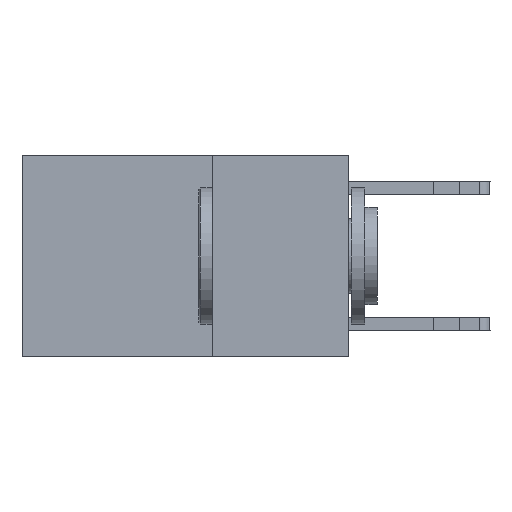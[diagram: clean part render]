
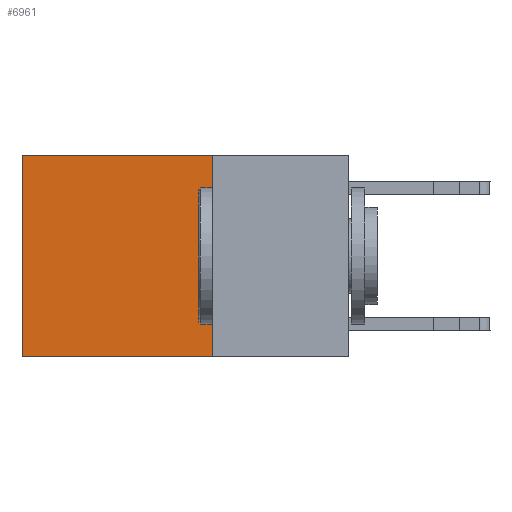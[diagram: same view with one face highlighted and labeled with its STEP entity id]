
A CAD part, left-side view. The second image highlights one B-rep face of the part: STEP entity #6961.
In plain terms, the highlighted planar face has unit normal (-1, 0, 0).
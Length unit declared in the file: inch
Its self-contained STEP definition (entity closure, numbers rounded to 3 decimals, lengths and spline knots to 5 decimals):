
#176 = AXIS2_PLACEMENT_3D ( 'NONE', #13911, #6382, #18770 ) ;
#232 = DIRECTION ( 'NONE',  ( 0., 0., -1. ) ) ;
#1264 = LINE ( 'NONE', #7343, #15404 ) ;
#1530 = LINE ( 'NONE', #12362, #6973 ) ;
#3976 = CARTESIAN_POINT ( 'NONE',  ( 0.2625, 0.6, 0. ) ) ;
#4156 = DIRECTION ( 'NONE',  ( 0., 1., 0. ) ) ;
#4174 = DIRECTION ( 'NONE',  ( 0., 0., -1. ) ) ;
#4298 = VERTEX_POINT ( 'NONE', #5183 ) ;
#4659 = ORIENTED_EDGE ( 'NONE', *, *, #18073, .F. ) ;
#5048 = CARTESIAN_POINT ( 'NONE',  ( 0.2625, 0.25, -0.37 ) ) ;
#5183 = CARTESIAN_POINT ( 'NONE',  ( 0.2625, 0.6, -0.37 ) ) ;
#6025 = CARTESIAN_POINT ( 'NONE',  ( 0.2625, 0.25, -0.37 ) ) ;
#6382 = DIRECTION ( 'NONE',  ( 1., 0., 0. ) ) ;
#6961 = ADVANCED_FACE ( 'NONE', ( #7969 ), #11144, .F. ) ;
#6973 = VECTOR ( 'NONE', #232, 39.37008 ) ;
#7343 = CARTESIAN_POINT ( 'NONE',  ( 0.2625, 0.25, 0. ) ) ;
#7389 = EDGE_CURVE ( 'NONE', #13159, #4298, #8131, .T. ) ;
#7969 = FACE_OUTER_BOUND ( 'NONE', #15587, .T. ) ;
#8131 = LINE ( 'NONE', #5048, #16629 ) ;
#8280 = CARTESIAN_POINT ( 'NONE',  ( 0.2625, 0.25, 0. ) ) ;
#8467 = EDGE_CURVE ( 'NONE', #16911, #15766, #1264, .T. ) ;
#8941 = LINE ( 'NONE', #10148, #17370 ) ;
#10148 = CARTESIAN_POINT ( 'NONE',  ( 0.2625, 0.6, 0. ) ) ;
#11144 = PLANE ( 'NONE',  #176 ) ;
#12058 = ORIENTED_EDGE ( 'NONE', *, *, #7389, .F. ) ;
#12362 = CARTESIAN_POINT ( 'NONE',  ( 0.2625, 0.25, 0. ) ) ;
#13159 = VERTEX_POINT ( 'NONE', #6025 ) ;
#13911 = CARTESIAN_POINT ( 'NONE',  ( 0.2625, 0.25, 0. ) ) ;
#15404 = VECTOR ( 'NONE', #4156, 39.37008 ) ;
#15467 = DIRECTION ( 'NONE',  ( 0., 1., 0. ) ) ;
#15587 = EDGE_LOOP ( 'NONE', ( #16062, #12058, #4659, #17734 ) ) ;
#15766 = VERTEX_POINT ( 'NONE', #3976 ) ;
#16062 = ORIENTED_EDGE ( 'NONE', *, *, #17173, .T. ) ;
#16629 = VECTOR ( 'NONE', #15467, 39.37008 ) ;
#16911 = VERTEX_POINT ( 'NONE', #8280 ) ;
#17173 = EDGE_CURVE ( 'NONE', #15766, #4298, #8941, .T. ) ;
#17370 = VECTOR ( 'NONE', #4174, 39.37008 ) ;
#17734 = ORIENTED_EDGE ( 'NONE', *, *, #8467, .T. ) ;
#18073 = EDGE_CURVE ( 'NONE', #16911, #13159, #1530, .T. ) ;
#18770 = DIRECTION ( 'NONE',  ( 0., 0., -1. ) ) ;
